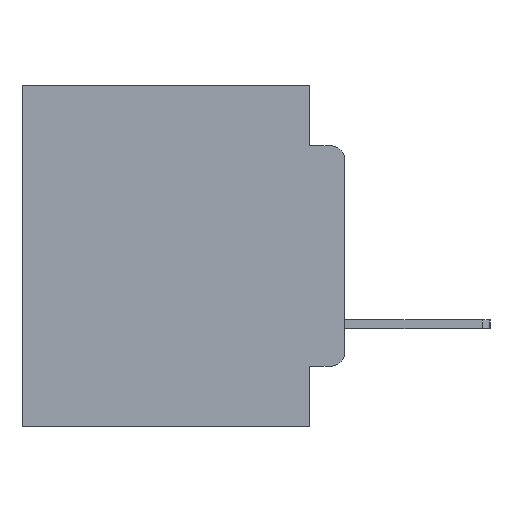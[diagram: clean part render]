
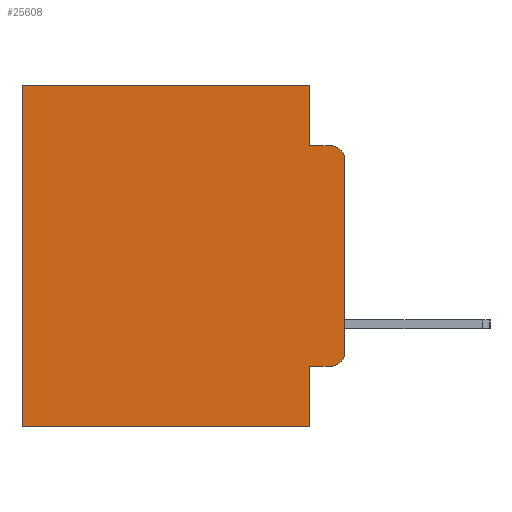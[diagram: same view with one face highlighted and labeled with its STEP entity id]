
A CAD part, left-side view. The second image highlights one B-rep face of the part: STEP entity #25608.
In plain terms, the highlighted planar face has unit normal (-1, 0, 0).
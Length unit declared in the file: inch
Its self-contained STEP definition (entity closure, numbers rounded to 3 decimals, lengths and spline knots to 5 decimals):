
#352 = VERTEX_POINT ( 'NONE', #14353 ) ;
#446 = DIRECTION ( 'NONE',  ( 0., 0., -1. ) ) ;
#813 = VERTEX_POINT ( 'NONE', #22895 ) ;
#912 = CARTESIAN_POINT ( 'NONE',  ( 0.298, 0.051, -0.4115 ) ) ;
#1276 = CARTESIAN_POINT ( 'NONE',  ( 0.298, 0., 0. ) ) ;
#2528 = AXIS2_PLACEMENT_3D ( 'NONE', #15891, #3706, #17853 ) ;
#3444 = ORIENTED_EDGE ( 'NONE', *, *, #14130, .T. ) ;
#3706 = DIRECTION ( 'NONE',  ( -1., 0., 0. ) ) ;
#4192 = VERTEX_POINT ( 'NONE', #11708 ) ;
#4700 = VERTEX_POINT ( 'NONE', #23063 ) ;
#5328 = AXIS2_PLACEMENT_3D ( 'NONE', #24422, #12762, #446 ) ;
#5391 = DIRECTION ( 'NONE',  ( 0., 0., -1. ) ) ;
#5800 = DIRECTION ( 'NONE',  ( 0., 0., -1. ) ) ;
#5822 = VERTEX_POINT ( 'NONE', #16856 ) ;
#8319 = ORIENTED_EDGE ( 'NONE', *, *, #8915, .T. ) ;
#8418 = VECTOR ( 'NONE', #17042, 39.37008 ) ;
#8630 = CARTESIAN_POINT ( 'NONE',  ( 0.298, 0., -0.5 ) ) ;
#8721 = EDGE_CURVE ( 'NONE', #5822, #813, #21550, .T. ) ;
#8854 = VECTOR ( 'NONE', #24402, 39.37008 ) ;
#8915 = EDGE_CURVE ( 'NONE', #11232, #21959, #16623, .T. ) ;
#8964 = ORIENTED_EDGE ( 'NONE', *, *, #17073, .F. ) ;
#9476 = CARTESIAN_POINT ( 'NONE',  ( 0.298, 0.051, -0.4115 ) ) ;
#10110 = EDGE_CURVE ( 'NONE', #24453, #5822, #24763, .T. ) ;
#11140 = AXIS2_PLACEMENT_3D ( 'NONE', #1276, #17475, #5391 ) ;
#11223 = ORIENTED_EDGE ( 'NONE', *, *, #24581, .F. ) ;
#11232 = VERTEX_POINT ( 'NONE', #22818 ) ;
#11384 = LINE ( 'NONE', #19772, #21228 ) ;
#11486 = EDGE_CURVE ( 'NONE', #24453, #4192, #12493, .T. ) ;
#11626 = CARTESIAN_POINT ( 'NONE',  ( 0.298, 0., -0.1085 ) ) ;
#11708 = CARTESIAN_POINT ( 'NONE',  ( 0.298, 0.051, -0.5 ) ) ;
#11769 = VECTOR ( 'NONE', #23327, 39.37008 ) ;
#12401 = CARTESIAN_POINT ( 'NONE',  ( 0.298, 0.473, 0. ) ) ;
#12448 = CARTESIAN_POINT ( 'NONE',  ( 0.298, 0., 0. ) ) ;
#12493 = LINE ( 'NONE', #13823, #17068 ) ;
#12762 = DIRECTION ( 'NONE',  ( -1., 0., 0. ) ) ;
#13554 = PLANE ( 'NONE',  #11140 ) ;
#13823 = CARTESIAN_POINT ( 'NONE',  ( 0.298, 0.051, 0. ) ) ;
#14130 = EDGE_CURVE ( 'NONE', #21959, #4700, #19240, .T. ) ;
#14171 = CIRCLE ( 'NONE', #5328, 0.02 ) ;
#14216 = LINE ( 'NONE', #8630, #8854 ) ;
#14353 = CARTESIAN_POINT ( 'NONE',  ( 0.298, 0.02, -0.0885 ) ) ;
#14375 = DIRECTION ( 'NONE',  ( 0., 0., -1. ) ) ;
#14461 = VERTEX_POINT ( 'NONE', #17338 ) ;
#14657 = VECTOR ( 'NONE', #14375, 39.37008 ) ;
#15459 = EDGE_CURVE ( 'NONE', #11232, #14461, #18567, .T. ) ;
#15568 = ORIENTED_EDGE ( 'NONE', *, *, #8721, .T. ) ;
#15891 = CARTESIAN_POINT ( 'NONE',  ( 0.298, 0.02, -0.3915 ) ) ;
#16021 = VECTOR ( 'NONE', #16394, 39.37008 ) ;
#16394 = DIRECTION ( 'NONE',  ( 0., 1., 0. ) ) ;
#16623 = LINE ( 'NONE', #12448, #16021 ) ;
#16762 = EDGE_CURVE ( 'NONE', #14461, #352, #22201, .T. ) ;
#16853 = FACE_OUTER_BOUND ( 'NONE', #22281, .T. ) ;
#16856 = CARTESIAN_POINT ( 'NONE',  ( 0.298, 0.02, -0.4115 ) ) ;
#17042 = DIRECTION ( 'NONE',  ( 0., -1., 0. ) ) ;
#17057 = ORIENTED_EDGE ( 'NONE', *, *, #16762, .F. ) ;
#17068 = VECTOR ( 'NONE', #17678, 39.37008 ) ;
#17073 = EDGE_CURVE ( 'NONE', #4192, #4700, #14216, .T. ) ;
#17318 = VECTOR ( 'NONE', #19314, 39.37008 ) ;
#17333 = CARTESIAN_POINT ( 'NONE',  ( 0.298, 0.051, 0. ) ) ;
#17338 = CARTESIAN_POINT ( 'NONE',  ( 0.298, 0.051, -0.0885 ) ) ;
#17475 = DIRECTION ( 'NONE',  ( 1., 0., 0. ) ) ;
#17678 = DIRECTION ( 'NONE',  ( 0., 0., -1. ) ) ;
#17853 = DIRECTION ( 'NONE',  ( 0., 0., -1. ) ) ;
#18310 = ORIENTED_EDGE ( 'NONE', *, *, #15459, .F. ) ;
#18324 = CARTESIAN_POINT ( 'NONE',  ( 0.298, 0.473, 0. ) ) ;
#18567 = LINE ( 'NONE', #17333, #17318 ) ;
#19114 = VERTEX_POINT ( 'NONE', #11626 ) ;
#19240 = LINE ( 'NONE', #12401, #14657 ) ;
#19314 = DIRECTION ( 'NONE',  ( 0., 0., -1. ) ) ;
#19531 = ORIENTED_EDGE ( 'NONE', *, *, #11486, .F. ) ;
#19772 = CARTESIAN_POINT ( 'NONE',  ( 0.298, 0., 0. ) ) ;
#21228 = VECTOR ( 'NONE', #5800, 39.37008 ) ;
#21407 = CARTESIAN_POINT ( 'NONE',  ( 0.298, 0.051, -0.0885 ) ) ;
#21550 = CIRCLE ( 'NONE', #2528, 0.02 ) ;
#21676 = ORIENTED_EDGE ( 'NONE', *, *, #22016, .T. ) ;
#21959 = VERTEX_POINT ( 'NONE', #18324 ) ;
#22016 = EDGE_CURVE ( 'NONE', #19114, #352, #14171, .T. ) ;
#22201 = LINE ( 'NONE', #21407, #11769 ) ;
#22281 = EDGE_LOOP ( 'NONE', ( #11223, #21676, #17057, #18310, #8319, #3444, #8964, #19531, #25293, #15568 ) ) ;
#22818 = CARTESIAN_POINT ( 'NONE',  ( 0.298, 0.051, 0. ) ) ;
#22895 = CARTESIAN_POINT ( 'NONE',  ( 0.298, 0., -0.3915 ) ) ;
#23063 = CARTESIAN_POINT ( 'NONE',  ( 0.298, 0.473, -0.5 ) ) ;
#23327 = DIRECTION ( 'NONE',  ( 0., -1., 0. ) ) ;
#24402 = DIRECTION ( 'NONE',  ( 0., 1., 0. ) ) ;
#24422 = CARTESIAN_POINT ( 'NONE',  ( 0.298, 0.02, -0.1085 ) ) ;
#24453 = VERTEX_POINT ( 'NONE', #9476 ) ;
#24581 = EDGE_CURVE ( 'NONE', #19114, #813, #11384, .T. ) ;
#24763 = LINE ( 'NONE', #912, #8418 ) ;
#25293 = ORIENTED_EDGE ( 'NONE', *, *, #10110, .T. ) ;
#25608 = ADVANCED_FACE ( 'NONE', ( #16853 ), #13554, .F. ) ;
